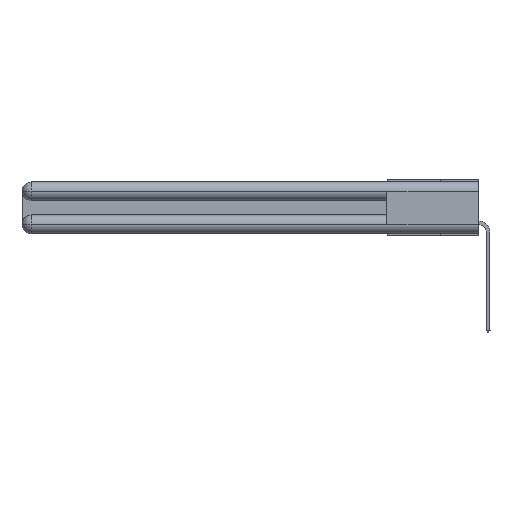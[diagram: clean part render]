
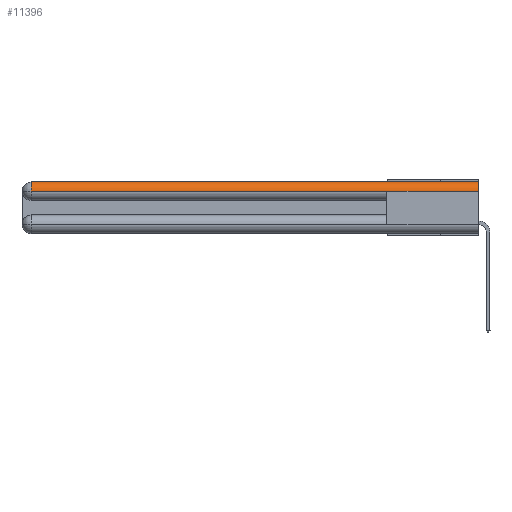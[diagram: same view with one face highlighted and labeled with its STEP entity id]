
A CAD part, left-side view. The second image highlights one B-rep face of the part: STEP entity #11396.
In plain terms, the highlighted cylindrical face has radius 1.562 mm (diameter 3.124 mm), a partial arc.
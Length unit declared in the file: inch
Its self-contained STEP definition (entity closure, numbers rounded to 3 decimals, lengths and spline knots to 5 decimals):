
#464 = VERTEX_POINT ( 'NONE', #9289 ) ;
#847 = DIRECTION ( 'NONE',  ( 0., -1., 0. ) ) ;
#1901 = EDGE_CURVE ( 'NONE', #5116, #2631, #11061, .T. ) ;
#2256 = CARTESIAN_POINT ( 'NONE',  ( 0., 0., -0.0615 ) ) ;
#2631 = VERTEX_POINT ( 'NONE', #8453 ) ;
#3572 = DIRECTION ( 'NONE',  ( 0., -1., 0. ) ) ;
#4275 = DIRECTION ( 'NONE',  ( 1., 0., 0. ) ) ;
#4474 = VERTEX_POINT ( 'NONE', #14597 ) ;
#4550 = DIRECTION ( 'NONE',  ( 0., 1., 0. ) ) ;
#5116 = VERTEX_POINT ( 'NONE', #7710 ) ;
#5884 = CIRCLE ( 'NONE', #25759, 0.0615 ) ;
#6845 = DIRECTION ( 'NONE',  ( 0., 0., 1. ) ) ;
#6865 = ORIENTED_EDGE ( 'NONE', *, *, #14456, .F. ) ;
#7710 = CARTESIAN_POINT ( 'NONE',  ( 0.0615, 2.94, 0. ) ) ;
#8453 = CARTESIAN_POINT ( 'NONE',  ( 0., 2.94, -0.0615 ) ) ;
#8983 = LINE ( 'NONE', #15987, #25662 ) ;
#9289 = CARTESIAN_POINT ( 'NONE',  ( 0., 0.6, -0.0615 ) ) ;
#9309 = EDGE_CURVE ( 'NONE', #2631, #464, #8983, .T. ) ;
#11043 = LINE ( 'NONE', #22685, #15273 ) ;
#11061 = CIRCLE ( 'NONE', #25959, 0.0615 ) ;
#11396 = ADVANCED_FACE ( 'NONE', ( #19440 ), #19096, .T. ) ;
#11509 = DIRECTION ( 'NONE',  ( 0., 0., 1. ) ) ;
#12130 = ORIENTED_EDGE ( 'NONE', *, *, #1901, .T. ) ;
#13584 = VERTEX_POINT ( 'NONE', #2256 ) ;
#14456 = EDGE_CURVE ( 'NONE', #4474, #13584, #5884, .T. ) ;
#14597 = CARTESIAN_POINT ( 'NONE',  ( 0.0615, 0., 0. ) ) ;
#15273 = VECTOR ( 'NONE', #18622, 39.37008 ) ;
#15987 = CARTESIAN_POINT ( 'NONE',  ( 0., 3., -0.0615 ) ) ;
#16763 = DIRECTION ( 'NONE',  ( 0., -1., 0. ) ) ;
#16858 = EDGE_CURVE ( 'NONE', #5116, #4474, #19651, .T. ) ;
#18622 = DIRECTION ( 'NONE',  ( 0., 1., 0. ) ) ;
#18943 = EDGE_LOOP ( 'NONE', ( #22969, #12130, #21505, #22481, #6865 ) ) ;
#19096 = CYLINDRICAL_SURFACE ( 'NONE', #25532, 0.0615 ) ;
#19174 = CARTESIAN_POINT ( 'NONE',  ( 0.0615, 0., -0.0615 ) ) ;
#19440 = FACE_OUTER_BOUND ( 'NONE', #18943, .T. ) ;
#19641 = CARTESIAN_POINT ( 'NONE',  ( 0.0615, 2.94, -0.0615 ) ) ;
#19651 = LINE ( 'NONE', #20443, #23283 ) ;
#20443 = CARTESIAN_POINT ( 'NONE',  ( 0.0615, 0., 0. ) ) ;
#20587 = EDGE_CURVE ( 'NONE', #13584, #464, #11043, .T. ) ;
#21363 = CARTESIAN_POINT ( 'NONE',  ( 0.0615, 0., -0.0615 ) ) ;
#21505 = ORIENTED_EDGE ( 'NONE', *, *, #9309, .T. ) ;
#22481 = ORIENTED_EDGE ( 'NONE', *, *, #20587, .F. ) ;
#22659 = DIRECTION ( 'NONE',  ( 0., -1., 0. ) ) ;
#22685 = CARTESIAN_POINT ( 'NONE',  ( 0., 3., -0.0615 ) ) ;
#22969 = ORIENTED_EDGE ( 'NONE', *, *, #16858, .F. ) ;
#23283 = VECTOR ( 'NONE', #22659, 39.37008 ) ;
#25532 = AXIS2_PLACEMENT_3D ( 'NONE', #21363, #4550, #6845 ) ;
#25662 = VECTOR ( 'NONE', #3572, 39.37008 ) ;
#25759 = AXIS2_PLACEMENT_3D ( 'NONE', #19174, #16763, #4275 ) ;
#25959 = AXIS2_PLACEMENT_3D ( 'NONE', #19641, #847, #11509 ) ;
